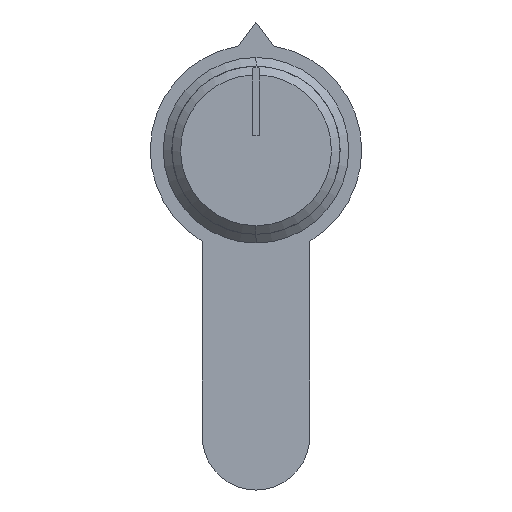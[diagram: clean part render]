
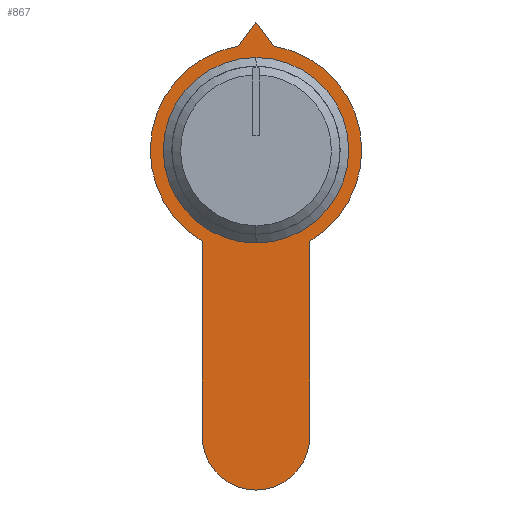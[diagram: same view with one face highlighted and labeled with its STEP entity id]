
A CAD part, left-side view. The second image highlights one B-rep face of the part: STEP entity #867.
In plain terms, the highlighted planar face has unit normal (-1, 0, 0).
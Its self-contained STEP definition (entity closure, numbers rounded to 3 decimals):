
#15 = CARTESIAN_POINT ( 'NONE',  ( 24., 0., 0. ) ) ;
#60 = AXIS2_PLACEMENT_3D ( 'NONE', #1410, #1859, #387 ) ;
#70 = CARTESIAN_POINT ( 'NONE',  ( 24., 3.1, -16.5 ) ) ;
#75 = AXIS2_PLACEMENT_3D ( 'NONE', #15, #752, #2474 ) ;
#136 = DIRECTION ( 'NONE',  ( 0., 0., -1. ) ) ;
#188 = EDGE_CURVE ( 'NONE', #1289, #1718, #3218, .T. ) ;
#192 = EDGE_CURVE ( 'NONE', #1458, #1800, #1664, .T. ) ;
#208 = VECTOR ( 'NONE', #3213, 1000. ) ;
#260 = AXIS2_PLACEMENT_3D ( 'NONE', #449, #972, #2473 ) ;
#262 = AXIS2_PLACEMENT_3D ( 'NONE', #2354, #2609, #848 ) ;
#306 = FACE_BOUND ( 'NONE', #2023, .T. ) ;
#335 = ORIENTED_EDGE ( 'NONE', *, *, #996, .F. ) ;
#387 = DIRECTION ( 'NONE',  ( 0., 0., -1. ) ) ;
#406 = PLANE ( 'NONE',  #2906 ) ;
#409 = ORIENTED_EDGE ( 'NONE', *, *, #2689, .T. ) ;
#449 = CARTESIAN_POINT ( 'NONE',  ( 24., 0., 0. ) ) ;
#560 = LINE ( 'NONE', #2482, #208 ) ;
#565 = VERTEX_POINT ( 'NONE', #2858 ) ;
#643 = DIRECTION ( 'NONE',  ( 1., 0., 0. ) ) ;
#752 = DIRECTION ( 'NONE',  ( 1., 0., 0. ) ) ;
#848 = DIRECTION ( 'NONE',  ( 0., 0., -1. ) ) ;
#867 = ADVANCED_FACE ( 'NONE', ( #306, #1798 ), #406, .F. ) ;
#873 = AXIS2_PLACEMENT_3D ( 'NONE', #1257, #2938, #1463 ) ;
#876 = VECTOR ( 'NONE', #1343, 1000. ) ;
#891 = CARTESIAN_POINT ( 'NONE',  ( 24., -3.1, 0. ) ) ;
#946 = EDGE_LOOP ( 'NONE', ( #1821, #335, #409, #2251, #2848, #1819, #2005 ) ) ;
#972 = DIRECTION ( 'NONE',  ( 1., 0., 0. ) ) ;
#979 = VERTEX_POINT ( 'NONE', #1746 ) ;
#996 = EDGE_CURVE ( 'NONE', #979, #2944, #2759, .T. ) ;
#1016 = EDGE_CURVE ( 'NONE', #1800, #1458, #2692, .T. ) ;
#1107 = LINE ( 'NONE', #891, #1848 ) ;
#1127 = VERTEX_POINT ( 'NONE', #1526 ) ;
#1257 = CARTESIAN_POINT ( 'NONE',  ( 24., 0., 0. ) ) ;
#1289 = VERTEX_POINT ( 'NONE', #3103 ) ;
#1343 = DIRECTION ( 'NONE',  ( 0., 0.586, -0.81 ) ) ;
#1352 = ORIENTED_EDGE ( 'NONE', *, *, #1016, .T. ) ;
#1410 = CARTESIAN_POINT ( 'NONE',  ( 24., 0., -16.5 ) ) ;
#1425 = CARTESIAN_POINT ( 'NONE',  ( 24., 1., 6.017 ) ) ;
#1458 = VERTEX_POINT ( 'NONE', #1946 ) ;
#1463 = DIRECTION ( 'NONE',  ( 0., 0., -1. ) ) ;
#1518 = DIRECTION ( 'NONE',  ( 0., -0.586, -0.81 ) ) ;
#1526 = CARTESIAN_POINT ( 'NONE',  ( 24., -3.1, -5.254 ) ) ;
#1546 = EDGE_CURVE ( 'NONE', #2944, #1127, #2673, .T. ) ;
#1664 = CIRCLE ( 'NONE', #873, 5.35 ) ;
#1718 = VERTEX_POINT ( 'NONE', #1425 ) ;
#1746 = CARTESIAN_POINT ( 'NONE',  ( 24., 0., 7.4 ) ) ;
#1798 = FACE_OUTER_BOUND ( 'NONE', #946, .T. ) ;
#1800 = VERTEX_POINT ( 'NONE', #2747 ) ;
#1819 = ORIENTED_EDGE ( 'NONE', *, *, #2756, .T. ) ;
#1821 = ORIENTED_EDGE ( 'NONE', *, *, #1546, .F. ) ;
#1848 = VECTOR ( 'NONE', #2878, 1000. ) ;
#1859 = DIRECTION ( 'NONE',  ( -1., 0., 0. ) ) ;
#1927 = CARTESIAN_POINT ( 'NONE',  ( 24., 0., 0. ) ) ;
#1939 = ORIENTED_EDGE ( 'NONE', *, *, #192, .T. ) ;
#1946 = CARTESIAN_POINT ( 'NONE',  ( 24., 0., -5.35 ) ) ;
#1961 = CARTESIAN_POINT ( 'NONE',  ( 24., -1., 6.017 ) ) ;
#1978 = CIRCLE ( 'NONE', #60, 3.1 ) ;
#2005 = ORIENTED_EDGE ( 'NONE', *, *, #2766, .F. ) ;
#2023 = EDGE_LOOP ( 'NONE', ( #1939, #1352 ) ) ;
#2056 = CARTESIAN_POINT ( 'NONE',  ( 24., 3.514, 2.542 ) ) ;
#2248 = VECTOR ( 'NONE', #1518, 1000. ) ;
#2251 = ORIENTED_EDGE ( 'NONE', *, *, #188, .F. ) ;
#2345 = LINE ( 'NONE', #2056, #876 ) ;
#2354 = CARTESIAN_POINT ( 'NONE',  ( 24., 0., 0. ) ) ;
#2473 = DIRECTION ( 'NONE',  ( 0., 0., -1. ) ) ;
#2474 = DIRECTION ( 'NONE',  ( 0., 0., -1. ) ) ;
#2482 = CARTESIAN_POINT ( 'NONE',  ( 24., 3.1, 0. ) ) ;
#2609 = DIRECTION ( 'NONE',  ( 1., 0., 0. ) ) ;
#2673 = CIRCLE ( 'NONE', #262, 6.1 ) ;
#2682 = VERTEX_POINT ( 'NONE', #70 ) ;
#2689 = EDGE_CURVE ( 'NONE', #979, #1718, #2345, .T. ) ;
#2692 = CIRCLE ( 'NONE', #75, 5.35 ) ;
#2747 = CARTESIAN_POINT ( 'NONE',  ( 24., 0., 5.35 ) ) ;
#2756 = EDGE_CURVE ( 'NONE', #2682, #565, #1978, .T. ) ;
#2759 = LINE ( 'NONE', #2995, #2248 ) ;
#2766 = EDGE_CURVE ( 'NONE', #1127, #565, #1107, .T. ) ;
#2848 = ORIENTED_EDGE ( 'NONE', *, *, #3041, .T. ) ;
#2858 = CARTESIAN_POINT ( 'NONE',  ( 24., -3.1, -16.5 ) ) ;
#2878 = DIRECTION ( 'NONE',  ( 0., 0., -1. ) ) ;
#2906 = AXIS2_PLACEMENT_3D ( 'NONE', #1927, #643, #136 ) ;
#2938 = DIRECTION ( 'NONE',  ( 1., 0., 0. ) ) ;
#2944 = VERTEX_POINT ( 'NONE', #1961 ) ;
#2995 = CARTESIAN_POINT ( 'NONE',  ( 24., -3.514, 2.542 ) ) ;
#3041 = EDGE_CURVE ( 'NONE', #1289, #2682, #560, .T. ) ;
#3103 = CARTESIAN_POINT ( 'NONE',  ( 24., 3.1, -5.254 ) ) ;
#3213 = DIRECTION ( 'NONE',  ( 0., 0., -1. ) ) ;
#3218 = CIRCLE ( 'NONE', #260, 6.1 ) ;
